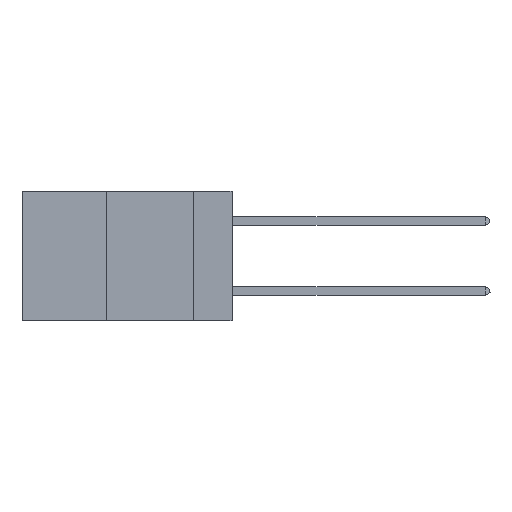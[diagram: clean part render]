
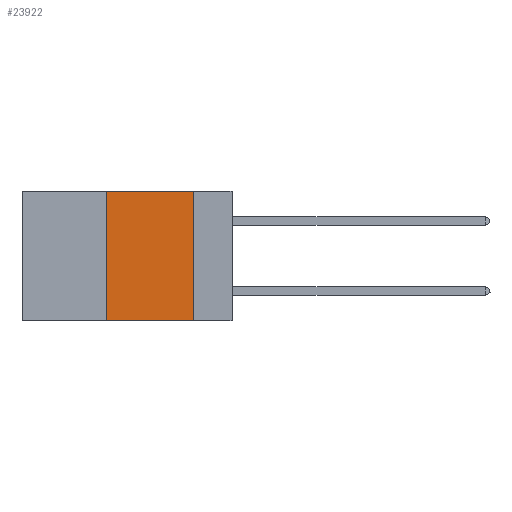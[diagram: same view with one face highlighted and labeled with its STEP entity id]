
A CAD part, left-side view. The second image highlights one B-rep face of the part: STEP entity #23922.
In plain terms, the highlighted planar face has unit normal (-1, 0, 0).
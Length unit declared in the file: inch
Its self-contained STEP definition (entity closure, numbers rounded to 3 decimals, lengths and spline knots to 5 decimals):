
#3070 = LINE ( 'NONE', #23356, #27295 ) ;
#3118 = VERTEX_POINT ( 'NONE', #5718 ) ;
#5023 = DIRECTION ( 'NONE',  ( 0., 0., -1. ) ) ;
#5718 = CARTESIAN_POINT ( 'NONE',  ( 0., 0.11, 0. ) ) ;
#5725 = CARTESIAN_POINT ( 'NONE',  ( 0., 0.36, -0.37 ) ) ;
#6530 = DIRECTION ( 'NONE',  ( 0., 0., -1. ) ) ;
#7555 = CARTESIAN_POINT ( 'NONE',  ( 0., 0.6, 0. ) ) ;
#8197 = LINE ( 'NONE', #14631, #34085 ) ;
#10506 = DIRECTION ( 'NONE',  ( 0., -1., 0. ) ) ;
#11959 = EDGE_CURVE ( 'NONE', #32944, #29913, #25023, .T. ) ;
#13704 = CARTESIAN_POINT ( 'NONE',  ( 0., 0.36, 0. ) ) ;
#14470 = AXIS2_PLACEMENT_3D ( 'NONE', #16245, #21874, #5023 ) ;
#14631 = CARTESIAN_POINT ( 'NONE',  ( 0., 0.6, -0.37 ) ) ;
#15532 = EDGE_LOOP ( 'NONE', ( #24372, #21377, #15707, #27199 ) ) ;
#15707 = ORIENTED_EDGE ( 'NONE', *, *, #11959, .F. ) ;
#16245 = CARTESIAN_POINT ( 'NONE',  ( 0., 0.6, 0. ) ) ;
#16408 = EDGE_CURVE ( 'NONE', #3118, #34434, #3070, .T. ) ;
#17015 = DIRECTION ( 'NONE',  ( 0., 0., 1. ) ) ;
#21080 = EDGE_CURVE ( 'NONE', #29913, #3118, #34231, .T. ) ;
#21377 = ORIENTED_EDGE ( 'NONE', *, *, #21080, .F. ) ;
#21874 = DIRECTION ( 'NONE',  ( 1., 0., 0. ) ) ;
#23356 = CARTESIAN_POINT ( 'NONE',  ( 0., 0.11, 0. ) ) ;
#23922 = ADVANCED_FACE ( 'NONE', ( #28469 ), #35728, .F. ) ;
#24372 = ORIENTED_EDGE ( 'NONE', *, *, #16408, .F. ) ;
#25023 = LINE ( 'NONE', #13704, #34678 ) ;
#25181 = EDGE_CURVE ( 'NONE', #32944, #34434, #8197, .T. ) ;
#25728 = CARTESIAN_POINT ( 'NONE',  ( 0., 0.36, 0. ) ) ;
#25889 = VECTOR ( 'NONE', #10506, 39.37008 ) ;
#25979 = CARTESIAN_POINT ( 'NONE',  ( 0., 0.11, -0.37 ) ) ;
#27199 = ORIENTED_EDGE ( 'NONE', *, *, #25181, .T. ) ;
#27295 = VECTOR ( 'NONE', #6530, 39.37008 ) ;
#28469 = FACE_OUTER_BOUND ( 'NONE', #15532, .T. ) ;
#29913 = VERTEX_POINT ( 'NONE', #25728 ) ;
#32944 = VERTEX_POINT ( 'NONE', #5725 ) ;
#34085 = VECTOR ( 'NONE', #34341, 39.37008 ) ;
#34231 = LINE ( 'NONE', #7555, #25889 ) ;
#34341 = DIRECTION ( 'NONE',  ( 0., -1., 0. ) ) ;
#34434 = VERTEX_POINT ( 'NONE', #25979 ) ;
#34678 = VECTOR ( 'NONE', #17015, 39.37008 ) ;
#35728 = PLANE ( 'NONE',  #14470 ) ;
